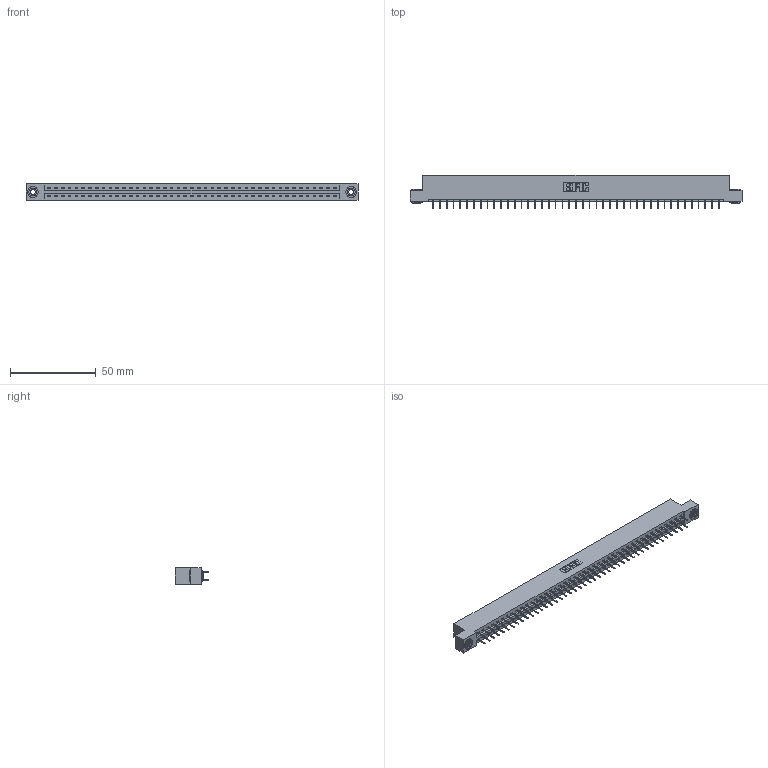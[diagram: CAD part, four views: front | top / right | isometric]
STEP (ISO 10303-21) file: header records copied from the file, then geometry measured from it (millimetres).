
FILE_DESCRIPTION (( 'STEP AP203' ), '1' );
FILE_NAME ('337-086-524-203.STEP', '2019-10-10T14:52:44', ( '' ), ( '' ), 'SwSTEP 2.0', 'SolidWorks 2016', '' );
FILE_SCHEMA (( 'CONFIG_CONTROL_DESIGN' ));
Length unit declared in the file: inch
Products named in the file (4): 337 Part_Flush Mounting Lugs - 0.156 Dia-TH; 345-250-002_345-250-002-102; 345-292-001_345-293-124; 337-086-524-203
Assembly tree (89 placements, depth 2):
  337-086-524-203
    337 Part_Flush Mounting Lugs - 0.156 Dia-TH
    345-292-001_345-293-124  x86
    345-250-002_345-250-002-102  x2
Bounding box: 193.4 x 19.69 x 9.4 mm (x, y, z)
Volume: 20284.1 mm3; surface area: 22762.3 mm2
Topology: 89 solids, 89 shells, 5140 faces, 14577 edges, 9370 vertices
Faces by surface type: plane 3864, cylinder 1268, cone 8
Entity records: 33934 total; most frequent: CARTESIAN_POINT 5689, ORIENTED_EDGE 5618, DIRECTION 4871, EDGE_CURVE 2809, LINE 2661, VECTOR 2661, VERTEX_POINT 1866, AXIS2_PLACEMENT_3D 1105
